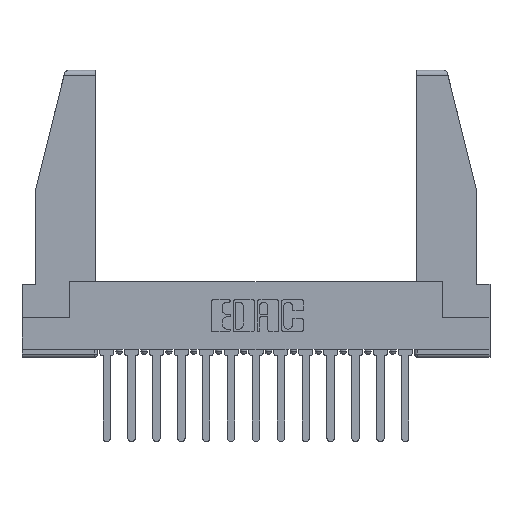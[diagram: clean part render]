
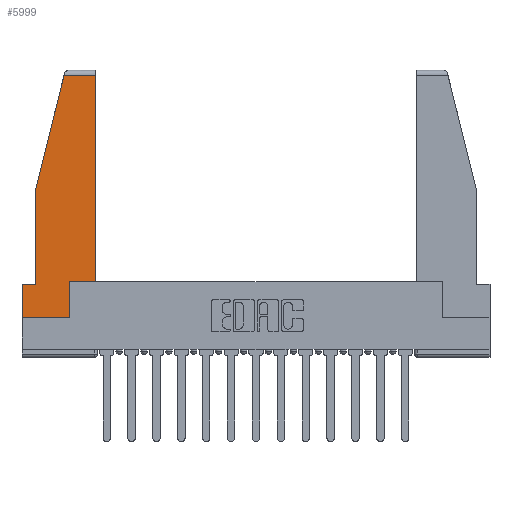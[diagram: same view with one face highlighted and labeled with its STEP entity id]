
A CAD part, top view. The second image highlights one B-rep face of the part: STEP entity #5999.
In plain terms, the highlighted planar face has unit normal (0, 0, 1).
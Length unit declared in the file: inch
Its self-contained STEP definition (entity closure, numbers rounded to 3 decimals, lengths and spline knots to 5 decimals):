
#53 = LINE ( 'NONE', #8701, #11762 ) ;
#264 = CARTESIAN_POINT ( 'NONE',  ( 0.2636, 1.52, 0. ) ) ;
#428 = ORIENTED_EDGE ( 'NONE', *, *, #15047, .T. ) ;
#774 = VECTOR ( 'NONE', #9510, 39.37008 ) ;
#1134 = LINE ( 'NONE', #14384, #9542 ) ;
#1177 = CARTESIAN_POINT ( 'NONE',  ( 0.297, 0.223, 0. ) ) ;
#1213 = LINE ( 'NONE', #16371, #13369 ) ;
#1253 = CARTESIAN_POINT ( 'NONE',  ( 0.086, 0.8, 0. ) ) ;
#1357 = VERTEX_POINT ( 'NONE', #7252 ) ;
#1438 = EDGE_CURVE ( 'NONE', #8243, #2198, #11738, .T. ) ;
#1525 = VECTOR ( 'NONE', #9186, 39.37008 ) ;
#2198 = VERTEX_POINT ( 'NONE', #264 ) ;
#2199 = VERTEX_POINT ( 'NONE', #5630 ) ;
#2274 = VECTOR ( 'NONE', #3326, 39.37008 ) ;
#2477 = CARTESIAN_POINT ( 'NONE',  ( 0.461, 0.223, 0. ) ) ;
#2643 = EDGE_CURVE ( 'NONE', #5834, #1357, #9020, .T. ) ;
#2740 = VERTEX_POINT ( 'NONE', #6605 ) ;
#2972 = EDGE_CURVE ( 'NONE', #2199, #5834, #11271, .T. ) ;
#2997 = CARTESIAN_POINT ( 'NONE',  ( 0.461, 1.52, 0. ) ) ;
#3311 = DIRECTION ( 'NONE',  ( -1., 0., 0. ) ) ;
#3326 = DIRECTION ( 'NONE',  ( 0., -1., 0. ) ) ;
#4467 = ORIENTED_EDGE ( 'NONE', *, *, #14873, .T. ) ;
#4580 = DIRECTION ( 'NONE',  ( -0.239, -0.971, 0. ) ) ;
#4726 = EDGE_CURVE ( 'NONE', #1357, #9326, #6179, .T. ) ;
#4736 = AXIS2_PLACEMENT_3D ( 'NONE', #15715, #16956, #15606 ) ;
#4772 = VECTOR ( 'NONE', #7838, 39.37008 ) ;
#4826 = VERTEX_POINT ( 'NONE', #16931 ) ;
#5420 = LINE ( 'NONE', #2477, #1525 ) ;
#5630 = CARTESIAN_POINT ( 'NONE',  ( 0.086, 0.8, 0. ) ) ;
#5733 = EDGE_CURVE ( 'NONE', #2740, #9060, #1213, .T. ) ;
#5834 = VERTEX_POINT ( 'NONE', #16434 ) ;
#5999 = ADVANCED_FACE ( 'NONE', ( #12926 ), #14245, .T. ) ;
#6179 = LINE ( 'NONE', #10107, #2274 ) ;
#6387 = VECTOR ( 'NONE', #3311, 39.37008 ) ;
#6605 = CARTESIAN_POINT ( 'NONE',  ( 0.297, 0., 0. ) ) ;
#7252 = CARTESIAN_POINT ( 'NONE',  ( 0., 0.21, 0. ) ) ;
#7838 = DIRECTION ( 'NONE',  ( 1., 0., 0. ) ) ;
#8243 = VERTEX_POINT ( 'NONE', #2997 ) ;
#8565 = DIRECTION ( 'NONE',  ( 0., 1., 0. ) ) ;
#8701 = CARTESIAN_POINT ( 'NONE',  ( 0.271, 1.55, 0. ) ) ;
#8959 = ORIENTED_EDGE ( 'NONE', *, *, #1438, .T. ) ;
#9020 = LINE ( 'NONE', #10134, #13384 ) ;
#9060 = VERTEX_POINT ( 'NONE', #13431 ) ;
#9128 = EDGE_LOOP ( 'NONE', ( #9563, #8959, #4467, #11508, #12004, #13608, #16972, #10139, #428 ) ) ;
#9186 = DIRECTION ( 'NONE',  ( 0., 1., 0. ) ) ;
#9275 = EDGE_CURVE ( 'NONE', #4826, #8243, #5420, .T. ) ;
#9326 = VERTEX_POINT ( 'NONE', #11778 ) ;
#9510 = DIRECTION ( 'NONE',  ( 0., -1., 0. ) ) ;
#9542 = VECTOR ( 'NONE', #10480, 39.37008 ) ;
#9563 = ORIENTED_EDGE ( 'NONE', *, *, #9275, .T. ) ;
#10107 = CARTESIAN_POINT ( 'NONE',  ( 0., 0.21, 0. ) ) ;
#10134 = CARTESIAN_POINT ( 'NONE',  ( 0., 0.21, 0. ) ) ;
#10139 = ORIENTED_EDGE ( 'NONE', *, *, #5733, .T. ) ;
#10480 = DIRECTION ( 'NONE',  ( 1., 0., 0. ) ) ;
#11271 = LINE ( 'NONE', #1253, #774 ) ;
#11508 = ORIENTED_EDGE ( 'NONE', *, *, #2972, .T. ) ;
#11738 = LINE ( 'NONE', #13803, #6387 ) ;
#11762 = VECTOR ( 'NONE', #4580, 39.37008 ) ;
#11778 = CARTESIAN_POINT ( 'NONE',  ( 0., 0., 0. ) ) ;
#12004 = ORIENTED_EDGE ( 'NONE', *, *, #2643, .T. ) ;
#12926 = FACE_OUTER_BOUND ( 'NONE', #9128, .T. ) ;
#13369 = VECTOR ( 'NONE', #8565, 39.37008 ) ;
#13384 = VECTOR ( 'NONE', #14250, 39.37008 ) ;
#13407 = EDGE_CURVE ( 'NONE', #9326, #2740, #1134, .T. ) ;
#13431 = CARTESIAN_POINT ( 'NONE',  ( 0.297, 0.223, 0. ) ) ;
#13608 = ORIENTED_EDGE ( 'NONE', *, *, #4726, .T. ) ;
#13803 = CARTESIAN_POINT ( 'NONE',  ( 0., 1.52, 0. ) ) ;
#14059 = LINE ( 'NONE', #1177, #4772 ) ;
#14245 = PLANE ( 'NONE',  #4736 ) ;
#14250 = DIRECTION ( 'NONE',  ( -1., 0., 0. ) ) ;
#14384 = CARTESIAN_POINT ( 'NONE',  ( 0., 0., 0. ) ) ;
#14873 = EDGE_CURVE ( 'NONE', #2198, #2199, #53, .T. ) ;
#15047 = EDGE_CURVE ( 'NONE', #9060, #4826, #14059, .T. ) ;
#15606 = DIRECTION ( 'NONE',  ( 1., 0., 0. ) ) ;
#15715 = CARTESIAN_POINT ( 'NONE',  ( 0., 0., 0. ) ) ;
#16371 = CARTESIAN_POINT ( 'NONE',  ( 0.297, 0., 0. ) ) ;
#16434 = CARTESIAN_POINT ( 'NONE',  ( 0.086, 0.21, 0. ) ) ;
#16931 = CARTESIAN_POINT ( 'NONE',  ( 0.461, 0.223, 0. ) ) ;
#16956 = DIRECTION ( 'NONE',  ( 0., 0., 1. ) ) ;
#16972 = ORIENTED_EDGE ( 'NONE', *, *, #13407, .T. ) ;
